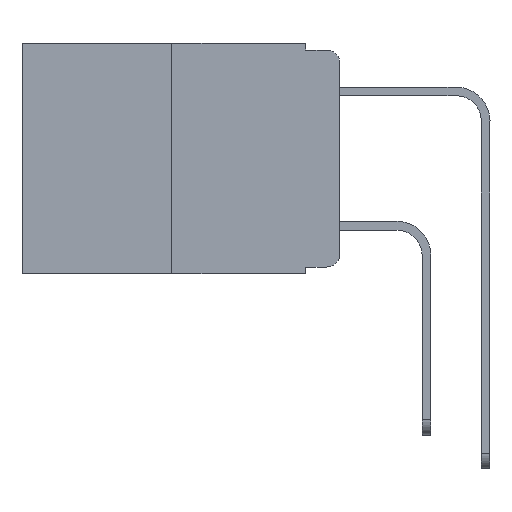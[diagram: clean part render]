
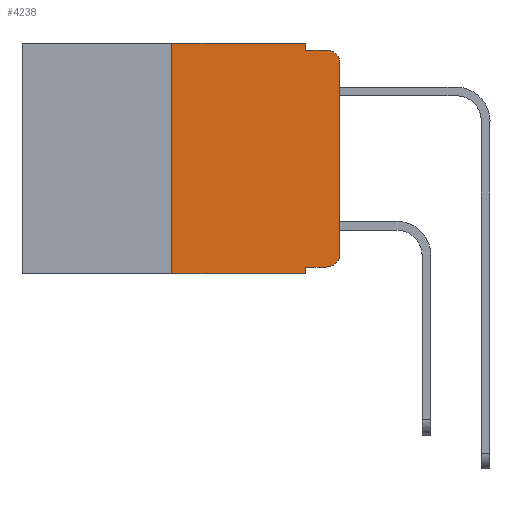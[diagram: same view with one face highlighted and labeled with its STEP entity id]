
A CAD part, left-side view. The second image highlights one B-rep face of the part: STEP entity #4238.
In plain terms, the highlighted planar face has unit normal (-1, 0, 0).
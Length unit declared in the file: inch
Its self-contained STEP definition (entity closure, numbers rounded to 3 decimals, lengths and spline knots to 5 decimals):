
#26 = ORIENTED_EDGE ( 'NONE', *, *, #1224, .T. ) ;
#970 = VECTOR ( 'NONE', #1362, 39.37008 ) ;
#1012 = VERTEX_POINT ( 'NONE', #4910 ) ;
#1206 = ORIENTED_EDGE ( 'NONE', *, *, #2568, .F. ) ;
#1224 = EDGE_CURVE ( 'NONE', #1922, #9611, #7428, .T. ) ;
#1356 = CARTESIAN_POINT ( 'NONE',  ( 0., 0.473, 0. ) ) ;
#1362 = DIRECTION ( 'NONE',  ( 0., -1., 0. ) ) ;
#1458 = CARTESIAN_POINT ( 'NONE',  ( 0., 0.051, -0.343 ) ) ;
#1523 = VECTOR ( 'NONE', #6862, 39.37008 ) ;
#1848 = AXIS2_PLACEMENT_3D ( 'NONE', #8508, #9989, #9876 ) ;
#1887 = ORIENTED_EDGE ( 'NONE', *, *, #2611, .T. ) ;
#1922 = VERTEX_POINT ( 'NONE', #10607 ) ;
#1949 = LINE ( 'NONE', #4460, #8735 ) ;
#2066 = CARTESIAN_POINT ( 'NONE',  ( 0., 0.051, -0.333 ) ) ;
#2496 = EDGE_CURVE ( 'NONE', #4271, #9904, #9738, .T. ) ;
#2568 = EDGE_CURVE ( 'NONE', #10221, #1012, #8066, .T. ) ;
#2611 = EDGE_CURVE ( 'NONE', #10938, #8542, #5366, .T. ) ;
#2614 = EDGE_CURVE ( 'NONE', #4271, #10938, #7804, .T. ) ;
#2633 = DIRECTION ( 'NONE',  ( 0., 0., 1. ) ) ;
#2675 = EDGE_CURVE ( 'NONE', #8542, #1922, #4204, .T. ) ;
#2697 = EDGE_CURVE ( 'NONE', #10416, #9611, #6275, .T. ) ;
#2771 = EDGE_CURVE ( 'NONE', #7356, #10416, #9943, .T. ) ;
#3717 = EDGE_LOOP ( 'NONE', ( #5241, #26, #7680, #5778, #6035, #1206, #3918, #10381, #8692, #1887 ) ) ;
#3918 = ORIENTED_EDGE ( 'NONE', *, *, #9922, .T. ) ;
#4204 = LINE ( 'NONE', #6921, #1523 ) ;
#4238 = ADVANCED_FACE ( 'NONE', ( #8519 ), #6225, .F. ) ;
#4259 = EDGE_CURVE ( 'NONE', #1012, #7356, #8285, .T. ) ;
#4271 = VERTEX_POINT ( 'NONE', #5431 ) ;
#4455 = CARTESIAN_POINT ( 'NONE',  ( 0., 0.02, -0.333 ) ) ;
#4460 = CARTESIAN_POINT ( 'NONE',  ( 0., 0.473, -0.343 ) ) ;
#4910 = CARTESIAN_POINT ( 'NONE',  ( 0., 0.25, 0. ) ) ;
#5048 = CARTESIAN_POINT ( 'NONE',  ( 0., 0.051, -0.01 ) ) ;
#5241 = ORIENTED_EDGE ( 'NONE', *, *, #2675, .T. ) ;
#5366 = CIRCLE ( 'NONE', #6902, 0.02 ) ;
#5431 = CARTESIAN_POINT ( 'NONE',  ( 0., 0.051, -0.333 ) ) ;
#5778 = ORIENTED_EDGE ( 'NONE', *, *, #2771, .F. ) ;
#6035 = ORIENTED_EDGE ( 'NONE', *, *, #4259, .F. ) ;
#6040 = DIRECTION ( 'NONE',  ( 0., 0., -1. ) ) ;
#6225 = PLANE ( 'NONE',  #1848 ) ;
#6275 = LINE ( 'NONE', #8624, #10154 ) ;
#6277 = DIRECTION ( 'NONE',  ( 0., 0., -1. ) ) ;
#6862 = DIRECTION ( 'NONE',  ( 0., 0., 1. ) ) ;
#6902 = AXIS2_PLACEMENT_3D ( 'NONE', #7287, #8581, #6040 ) ;
#6921 = CARTESIAN_POINT ( 'NONE',  ( 0., 0., 0. ) ) ;
#7247 = AXIS2_PLACEMENT_3D ( 'NONE', #10425, #8263, #8463 ) ;
#7287 = CARTESIAN_POINT ( 'NONE',  ( 0., 0.02, -0.313 ) ) ;
#7306 = CARTESIAN_POINT ( 'NONE',  ( 0., 0.25, -0.343 ) ) ;
#7356 = VERTEX_POINT ( 'NONE', #10391 ) ;
#7428 = CIRCLE ( 'NONE', #7247, 0.02 ) ;
#7680 = ORIENTED_EDGE ( 'NONE', *, *, #2697, .F. ) ;
#7804 = LINE ( 'NONE', #2066, #11229 ) ;
#7925 = VECTOR ( 'NONE', #6277, 39.37008 ) ;
#8066 = LINE ( 'NONE', #9729, #9842 ) ;
#8263 = DIRECTION ( 'NONE',  ( -1., 0., 0. ) ) ;
#8285 = LINE ( 'NONE', #1356, #970 ) ;
#8463 = DIRECTION ( 'NONE',  ( 0., 0., -1. ) ) ;
#8508 = CARTESIAN_POINT ( 'NONE',  ( 0., 0.473, 0. ) ) ;
#8519 = FACE_OUTER_BOUND ( 'NONE', #3717, .T. ) ;
#8542 = VERTEX_POINT ( 'NONE', #8868 ) ;
#8581 = DIRECTION ( 'NONE',  ( -1., 0., 0. ) ) ;
#8624 = CARTESIAN_POINT ( 'NONE',  ( 0., 0.051, -0.01 ) ) ;
#8646 = DIRECTION ( 'NONE',  ( 0., -1., 0. ) ) ;
#8678 = DIRECTION ( 'NONE',  ( 0., -1., 0. ) ) ;
#8692 = ORIENTED_EDGE ( 'NONE', *, *, #2614, .T. ) ;
#8735 = VECTOR ( 'NONE', #8678, 39.37008 ) ;
#8799 = VECTOR ( 'NONE', #9905, 39.37008 ) ;
#8868 = CARTESIAN_POINT ( 'NONE',  ( 0., 0., -0.313 ) ) ;
#9338 = CARTESIAN_POINT ( 'NONE',  ( 0., 0.051, 0. ) ) ;
#9611 = VERTEX_POINT ( 'NONE', #9879 ) ;
#9729 = CARTESIAN_POINT ( 'NONE',  ( 0., 0.25, 0. ) ) ;
#9738 = LINE ( 'NONE', #10015, #8799 ) ;
#9842 = VECTOR ( 'NONE', #2633, 39.37008 ) ;
#9876 = DIRECTION ( 'NONE',  ( 0., 0., -1. ) ) ;
#9879 = CARTESIAN_POINT ( 'NONE',  ( 0., 0.02, -0.01 ) ) ;
#9904 = VERTEX_POINT ( 'NONE', #1458 ) ;
#9905 = DIRECTION ( 'NONE',  ( 0., 0., -1. ) ) ;
#9922 = EDGE_CURVE ( 'NONE', #10221, #9904, #1949, .T. ) ;
#9943 = LINE ( 'NONE', #9338, #7925 ) ;
#9989 = DIRECTION ( 'NONE',  ( 1., 0., 0. ) ) ;
#10015 = CARTESIAN_POINT ( 'NONE',  ( 0., 0.051, 0. ) ) ;
#10154 = VECTOR ( 'NONE', #8646, 39.37008 ) ;
#10221 = VERTEX_POINT ( 'NONE', #7306 ) ;
#10381 = ORIENTED_EDGE ( 'NONE', *, *, #2496, .F. ) ;
#10391 = CARTESIAN_POINT ( 'NONE',  ( 0., 0.051, 0. ) ) ;
#10416 = VERTEX_POINT ( 'NONE', #5048 ) ;
#10425 = CARTESIAN_POINT ( 'NONE',  ( 0., 0.02, -0.03 ) ) ;
#10607 = CARTESIAN_POINT ( 'NONE',  ( 0., 0., -0.03 ) ) ;
#10938 = VERTEX_POINT ( 'NONE', #4455 ) ;
#11192 = DIRECTION ( 'NONE',  ( 0., -1., 0. ) ) ;
#11229 = VECTOR ( 'NONE', #11192, 39.37008 ) ;
